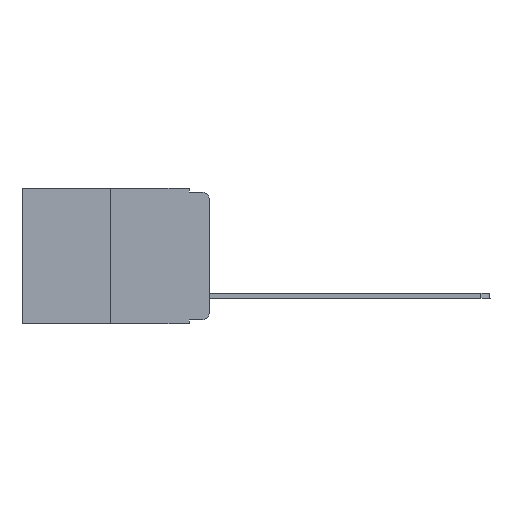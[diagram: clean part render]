
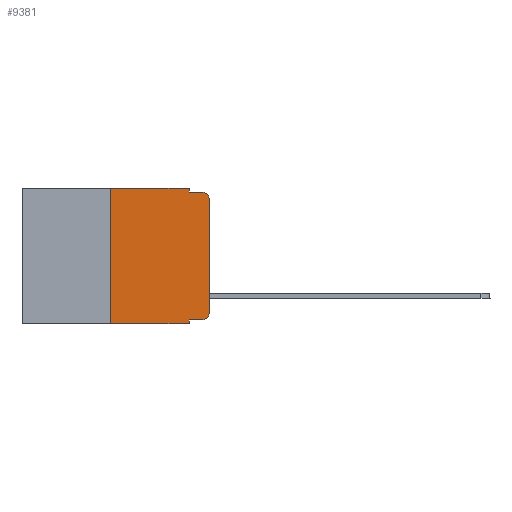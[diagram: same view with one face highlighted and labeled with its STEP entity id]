
A CAD part, left-side view. The second image highlights one B-rep face of the part: STEP entity #9381.
In plain terms, the highlighted planar face has unit normal (-1, 0, 0).
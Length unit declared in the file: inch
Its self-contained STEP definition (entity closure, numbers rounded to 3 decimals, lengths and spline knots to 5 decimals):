
#86 = CARTESIAN_POINT ( 'NONE',  ( 0., 0., -0.03 ) ) ;
#234 = CARTESIAN_POINT ( 'NONE',  ( 0., 0.02, -0.333 ) ) ;
#342 = CARTESIAN_POINT ( 'NONE',  ( 0., 0.051, 0. ) ) ;
#514 = EDGE_LOOP ( 'NONE', ( #1207, #12391, #5049, #2719, #11199, #6765, #11980, #5030, #7323, #8456 ) ) ;
#720 = CARTESIAN_POINT ( 'NONE',  ( 0., 0., 0. ) ) ;
#765 = VERTEX_POINT ( 'NONE', #86 ) ;
#1007 = CARTESIAN_POINT ( 'NONE',  ( 0., 0.473, 0. ) ) ;
#1199 = DIRECTION ( 'NONE',  ( 0., -1., 0. ) ) ;
#1207 = ORIENTED_EDGE ( 'NONE', *, *, #5251, .T. ) ;
#1342 = VERTEX_POINT ( 'NONE', #10638 ) ;
#1692 = DIRECTION ( 'NONE',  ( 0., 0., -1. ) ) ;
#1897 = LINE ( 'NONE', #6895, #3990 ) ;
#1903 = CIRCLE ( 'NONE', #10161, 0.02 ) ;
#1932 = VECTOR ( 'NONE', #9311, 39.37008 ) ;
#2039 = CARTESIAN_POINT ( 'NONE',  ( 0., 0.051, -0.01 ) ) ;
#2120 = VERTEX_POINT ( 'NONE', #10079 ) ;
#2682 = LINE ( 'NONE', #1007, #8728 ) ;
#2719 = ORIENTED_EDGE ( 'NONE', *, *, #4081, .F. ) ;
#2999 = EDGE_CURVE ( 'NONE', #5955, #9465, #10419, .T. ) ;
#3103 = DIRECTION ( 'NONE',  ( 0., -1., 0. ) ) ;
#3105 = DIRECTION ( 'NONE',  ( 0., 0., -1. ) ) ;
#3155 = AXIS2_PLACEMENT_3D ( 'NONE', #4793, #6957, #10924 ) ;
#3189 = CARTESIAN_POINT ( 'NONE',  ( 0., 0., -0.313 ) ) ;
#3616 = DIRECTION ( 'NONE',  ( 0., 0., 1. ) ) ;
#3633 = EDGE_CURVE ( 'NONE', #2120, #5501, #10100, .T. ) ;
#3882 = LINE ( 'NONE', #342, #5687 ) ;
#3990 = VECTOR ( 'NONE', #7911, 39.37008 ) ;
#4081 = EDGE_CURVE ( 'NONE', #8298, #2120, #3882, .T. ) ;
#4208 = DIRECTION ( 'NONE',  ( 0., 0., -1. ) ) ;
#4407 = CARTESIAN_POINT ( 'NONE',  ( 0., 0.051, -0.343 ) ) ;
#4543 = LINE ( 'NONE', #11108, #7696 ) ;
#4793 = CARTESIAN_POINT ( 'NONE',  ( 0., 0.02, -0.313 ) ) ;
#5030 = ORIENTED_EDGE ( 'NONE', *, *, #9082, .F. ) ;
#5049 = ORIENTED_EDGE ( 'NONE', *, *, #3633, .F. ) ;
#5159 = PLANE ( 'NONE',  #12352 ) ;
#5251 = EDGE_CURVE ( 'NONE', #9465, #765, #7408, .T. ) ;
#5501 = VERTEX_POINT ( 'NONE', #8926 ) ;
#5516 = CARTESIAN_POINT ( 'NONE',  ( 0., 0.25, -0.343 ) ) ;
#5663 = DIRECTION ( 'NONE',  ( 0., -1., 0. ) ) ;
#5687 = VECTOR ( 'NONE', #4208, 39.37008 ) ;
#5784 = EDGE_CURVE ( 'NONE', #11556, #8298, #2682, .T. ) ;
#5955 = VERTEX_POINT ( 'NONE', #234 ) ;
#6101 = DIRECTION ( 'NONE',  ( 1., 0., 0. ) ) ;
#6122 = LINE ( 'NONE', #8323, #1932 ) ;
#6146 = CARTESIAN_POINT ( 'NONE',  ( 0., 0.051, 0. ) ) ;
#6765 = ORIENTED_EDGE ( 'NONE', *, *, #8409, .F. ) ;
#6895 = CARTESIAN_POINT ( 'NONE',  ( 0., 0.051, -0.333 ) ) ;
#6957 = DIRECTION ( 'NONE',  ( -1., 0., 0. ) ) ;
#7323 = ORIENTED_EDGE ( 'NONE', *, *, #10469, .T. ) ;
#7408 = LINE ( 'NONE', #720, #11349 ) ;
#7600 = LINE ( 'NONE', #11396, #8526 ) ;
#7696 = VECTOR ( 'NONE', #1199, 39.37008 ) ;
#7911 = DIRECTION ( 'NONE',  ( 0., -1., 0. ) ) ;
#8069 = EDGE_CURVE ( 'NONE', #765, #5501, #1903, .T. ) ;
#8298 = VERTEX_POINT ( 'NONE', #6146 ) ;
#8323 = CARTESIAN_POINT ( 'NONE',  ( 0., 0.051, 0. ) ) ;
#8409 = EDGE_CURVE ( 'NONE', #10150, #11556, #7600, .T. ) ;
#8456 = ORIENTED_EDGE ( 'NONE', *, *, #2999, .T. ) ;
#8526 = VECTOR ( 'NONE', #3616, 39.37008 ) ;
#8728 = VECTOR ( 'NONE', #5663, 39.37008 ) ;
#8919 = CARTESIAN_POINT ( 'NONE',  ( 0., 0.473, 0. ) ) ;
#8926 = CARTESIAN_POINT ( 'NONE',  ( 0., 0.02, -0.01 ) ) ;
#9082 = EDGE_CURVE ( 'NONE', #1342, #9515, #6122, .T. ) ;
#9292 = DIRECTION ( 'NONE',  ( 0., 0., 1. ) ) ;
#9311 = DIRECTION ( 'NONE',  ( 0., 0., -1. ) ) ;
#9325 = DIRECTION ( 'NONE',  ( -1., 0., 0. ) ) ;
#9368 = CARTESIAN_POINT ( 'NONE',  ( 0., 0.02, -0.03 ) ) ;
#9381 = ADVANCED_FACE ( 'NONE', ( #12322 ), #5159, .F. ) ;
#9465 = VERTEX_POINT ( 'NONE', #3189 ) ;
#9515 = VERTEX_POINT ( 'NONE', #4407 ) ;
#9950 = VECTOR ( 'NONE', #3103, 39.37008 ) ;
#10079 = CARTESIAN_POINT ( 'NONE',  ( 0., 0.051, -0.01 ) ) ;
#10100 = LINE ( 'NONE', #2039, #9950 ) ;
#10150 = VERTEX_POINT ( 'NONE', #5516 ) ;
#10161 = AXIS2_PLACEMENT_3D ( 'NONE', #9368, #9325, #1692 ) ;
#10419 = CIRCLE ( 'NONE', #3155, 0.02 ) ;
#10469 = EDGE_CURVE ( 'NONE', #1342, #5955, #1897, .T. ) ;
#10638 = CARTESIAN_POINT ( 'NONE',  ( 0., 0.051, -0.333 ) ) ;
#10924 = DIRECTION ( 'NONE',  ( 0., 0., -1. ) ) ;
#11108 = CARTESIAN_POINT ( 'NONE',  ( 0., 0.473, -0.343 ) ) ;
#11199 = ORIENTED_EDGE ( 'NONE', *, *, #5784, .F. ) ;
#11349 = VECTOR ( 'NONE', #9292, 39.37008 ) ;
#11396 = CARTESIAN_POINT ( 'NONE',  ( 0., 0.25, 0. ) ) ;
#11556 = VERTEX_POINT ( 'NONE', #12120 ) ;
#11980 = ORIENTED_EDGE ( 'NONE', *, *, #12044, .T. ) ;
#12044 = EDGE_CURVE ( 'NONE', #10150, #9515, #4543, .T. ) ;
#12120 = CARTESIAN_POINT ( 'NONE',  ( 0., 0.25, 0. ) ) ;
#12322 = FACE_OUTER_BOUND ( 'NONE', #514, .T. ) ;
#12352 = AXIS2_PLACEMENT_3D ( 'NONE', #8919, #6101, #3105 ) ;
#12391 = ORIENTED_EDGE ( 'NONE', *, *, #8069, .T. ) ;
